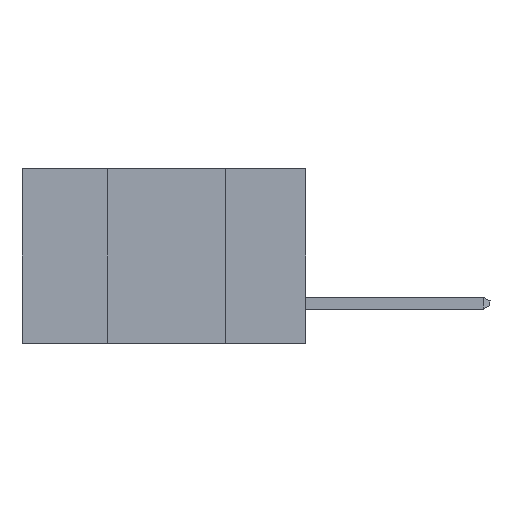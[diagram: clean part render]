
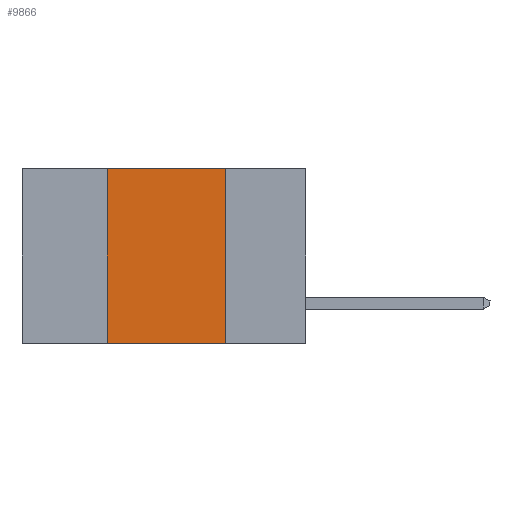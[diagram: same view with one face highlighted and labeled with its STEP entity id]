
A CAD part, left-side view. The second image highlights one B-rep face of the part: STEP entity #9866.
In plain terms, the highlighted planar face has unit normal (-1, 0, 0).
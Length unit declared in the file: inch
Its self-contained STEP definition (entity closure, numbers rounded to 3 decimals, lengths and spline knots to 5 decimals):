
#115 = CARTESIAN_POINT ( 'NONE',  ( 0., 0.17, -0.37 ) ) ;
#260 = CARTESIAN_POINT ( 'NONE',  ( 0., 0.42, 0. ) ) ;
#381 = EDGE_CURVE ( 'NONE', #9076, #7581, #5178, .T. ) ;
#639 = EDGE_CURVE ( 'NONE', #6715, #9076, #2968, .T. ) ;
#1501 = DIRECTION ( 'NONE',  ( 1., 0., 0. ) ) ;
#1772 = ORIENTED_EDGE ( 'NONE', *, *, #381, .F. ) ;
#1983 = EDGE_LOOP ( 'NONE', ( #1772, #2249, #4570, #10754 ) ) ;
#2249 = ORIENTED_EDGE ( 'NONE', *, *, #639, .F. ) ;
#2293 = VERTEX_POINT ( 'NONE', #4388 ) ;
#2826 = VECTOR ( 'NONE', #10623, 39.37008 ) ;
#2968 = LINE ( 'NONE', #5630, #10989 ) ;
#3598 = LINE ( 'NONE', #5380, #2826 ) ;
#3659 = CARTESIAN_POINT ( 'NONE',  ( 0., 0.6, -0.37 ) ) ;
#4085 = EDGE_CURVE ( 'NONE', #2293, #7581, #6265, .T. ) ;
#4223 = DIRECTION ( 'NONE',  ( 0., 0., -1. ) ) ;
#4239 = CARTESIAN_POINT ( 'NONE',  ( 0., 0.17, 0. ) ) ;
#4255 = FACE_OUTER_BOUND ( 'NONE', #1983, .T. ) ;
#4388 = CARTESIAN_POINT ( 'NONE',  ( 0., 0.42, -0.37 ) ) ;
#4570 = ORIENTED_EDGE ( 'NONE', *, *, #8362, .F. ) ;
#4606 = DIRECTION ( 'NONE',  ( 0., -1., 0. ) ) ;
#5053 = DIRECTION ( 'NONE',  ( 0., 0., -1. ) ) ;
#5178 = LINE ( 'NONE', #6897, #8633 ) ;
#5380 = CARTESIAN_POINT ( 'NONE',  ( 0., 0.42, -0.37 ) ) ;
#5561 = AXIS2_PLACEMENT_3D ( 'NONE', #9435, #1501, #5053 ) ;
#5630 = CARTESIAN_POINT ( 'NONE',  ( 0., 0.6, 0. ) ) ;
#6265 = LINE ( 'NONE', #3659, #8165 ) ;
#6715 = VERTEX_POINT ( 'NONE', #260 ) ;
#6897 = CARTESIAN_POINT ( 'NONE',  ( 0., 0.17, -0.37 ) ) ;
#6926 = PLANE ( 'NONE',  #5561 ) ;
#7581 = VERTEX_POINT ( 'NONE', #115 ) ;
#8165 = VECTOR ( 'NONE', #4606, 39.37008 ) ;
#8362 = EDGE_CURVE ( 'NONE', #2293, #6715, #3598, .T. ) ;
#8633 = VECTOR ( 'NONE', #4223, 39.37008 ) ;
#9076 = VERTEX_POINT ( 'NONE', #4239 ) ;
#9154 = DIRECTION ( 'NONE',  ( 0., -1., 0. ) ) ;
#9435 = CARTESIAN_POINT ( 'NONE',  ( 0., 0.6, 0. ) ) ;
#9866 = ADVANCED_FACE ( 'NONE', ( #4255 ), #6926, .F. ) ;
#10623 = DIRECTION ( 'NONE',  ( 0., 0., 1. ) ) ;
#10754 = ORIENTED_EDGE ( 'NONE', *, *, #4085, .T. ) ;
#10989 = VECTOR ( 'NONE', #9154, 39.37008 ) ;
